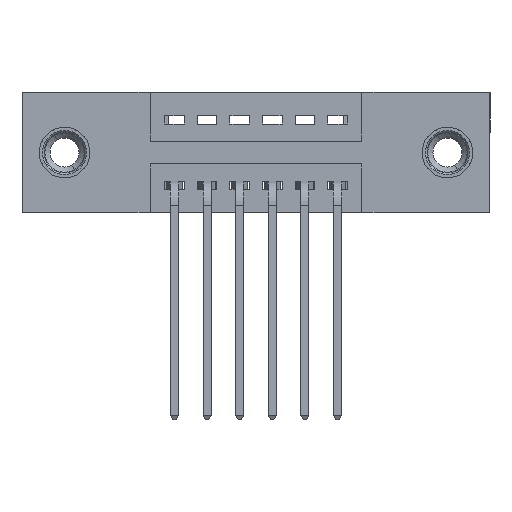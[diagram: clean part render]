
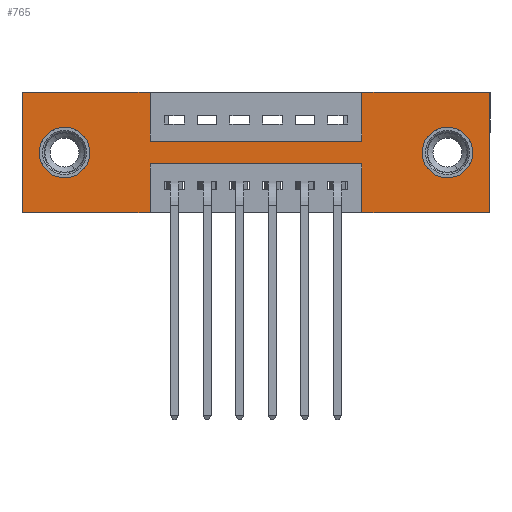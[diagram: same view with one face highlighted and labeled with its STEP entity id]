
A CAD part, front view. The second image highlights one B-rep face of the part: STEP entity #765.
In plain terms, the highlighted planar face has unit normal (0, -1, 0).
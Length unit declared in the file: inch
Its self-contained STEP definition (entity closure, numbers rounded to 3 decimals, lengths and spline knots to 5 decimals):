
#94 = EDGE_CURVE ( 'NONE', #12431, #1138, #12503, .T. ) ;
#183 = VECTOR ( 'NONE', #4928, 39.37008 ) ;
#296 = FACE_BOUND ( 'NONE', #9028, .T. ) ;
#588 = CIRCLE ( 'NONE', #4915, 0.078 ) ;
#644 = CARTESIAN_POINT ( 'NONE',  ( 0.13, 0., -0.107 ) ) ;
#658 = ORIENTED_EDGE ( 'NONE', *, *, #10039, .F. ) ;
#765 = ADVANCED_FACE ( 'NONE', ( #4771, #296, #13489 ), #11098, .T. ) ;
#838 = VERTEX_POINT ( 'NONE', #5530 ) ;
#1138 = VERTEX_POINT ( 'NONE', #4485 ) ;
#1227 = CARTESIAN_POINT ( 'NONE',  ( 0.3925, 0., -0.22 ) ) ;
#1370 = ORIENTED_EDGE ( 'NONE', *, *, #6849, .F. ) ;
#1428 = VECTOR ( 'NONE', #5903, 39.37008 ) ;
#1485 = VERTEX_POINT ( 'NONE', #1607 ) ;
#1607 = CARTESIAN_POINT ( 'NONE',  ( 0.3925, 0., -0.37 ) ) ;
#1695 = CARTESIAN_POINT ( 'NONE',  ( 0., 0., 0. ) ) ;
#1705 = LINE ( 'NONE', #1920, #8583 ) ;
#1823 = ORIENTED_EDGE ( 'NONE', *, *, #6230, .F. ) ;
#1887 = CARTESIAN_POINT ( 'NONE',  ( 0.13, 0., -0.185 ) ) ;
#1916 = ORIENTED_EDGE ( 'NONE', *, *, #2650, .T. ) ;
#1920 = CARTESIAN_POINT ( 'NONE',  ( 0.3925, 0., -0.15 ) ) ;
#1935 = VECTOR ( 'NONE', #2283, 39.37008 ) ;
#2012 = CARTESIAN_POINT ( 'NONE',  ( 0., 0., 0. ) ) ;
#2047 = CARTESIAN_POINT ( 'NONE',  ( 0.3925, 0., 0. ) ) ;
#2082 = CARTESIAN_POINT ( 'NONE',  ( 0., 0., 0. ) ) ;
#2233 = AXIS2_PLACEMENT_3D ( 'NONE', #7778, #4527, #12016 ) ;
#2283 = DIRECTION ( 'NONE',  ( 1., 0., 0. ) ) ;
#2321 = VECTOR ( 'NONE', #12269, 39.37008 ) ;
#2354 = VERTEX_POINT ( 'NONE', #5692 ) ;
#2363 = DIRECTION ( 'NONE',  ( -1., 0., 0. ) ) ;
#2560 = EDGE_LOOP ( 'NONE', ( #4301, #13436, #2651, #9678, #12162, #1823, #13720, #3026, #12351, #4077, #658, #1370 ) ) ;
#2614 = VERTEX_POINT ( 'NONE', #6707 ) ;
#2650 = EDGE_CURVE ( 'NONE', #10516, #6219, #588, .T. ) ;
#2651 = ORIENTED_EDGE ( 'NONE', *, *, #5780, .F. ) ;
#2665 = DIRECTION ( 'NONE',  ( 0., 0., 1. ) ) ;
#2971 = ORIENTED_EDGE ( 'NONE', *, *, #10768, .T. ) ;
#3026 = ORIENTED_EDGE ( 'NONE', *, *, #8182, .F. ) ;
#3046 = EDGE_CURVE ( 'NONE', #6951, #1485, #12585, .T. ) ;
#3249 = CARTESIAN_POINT ( 'NONE',  ( 0.3925, 0., -0.22 ) ) ;
#3559 = VERTEX_POINT ( 'NONE', #11444 ) ;
#3648 = LINE ( 'NONE', #7883, #11912 ) ;
#4024 = VERTEX_POINT ( 'NONE', #13758 ) ;
#4077 = ORIENTED_EDGE ( 'NONE', *, *, #7554, .F. ) ;
#4165 = CARTESIAN_POINT ( 'NONE',  ( 1.435, 0., 0. ) ) ;
#4234 = DIRECTION ( 'NONE',  ( 1., 0., 0. ) ) ;
#4301 = ORIENTED_EDGE ( 'NONE', *, *, #3046, .F. ) ;
#4451 = CARTESIAN_POINT ( 'NONE',  ( 1.305, 0., -0.107 ) ) ;
#4457 = VERTEX_POINT ( 'NONE', #2082 ) ;
#4485 = CARTESIAN_POINT ( 'NONE',  ( 0.13, 0., -0.263 ) ) ;
#4527 = DIRECTION ( 'NONE',  ( 0., -1., 0. ) ) ;
#4605 = CARTESIAN_POINT ( 'NONE',  ( 0., 0., 0. ) ) ;
#4749 = AXIS2_PLACEMENT_3D ( 'NONE', #12182, #8844, #5546 ) ;
#4771 = FACE_BOUND ( 'NONE', #10620, .T. ) ;
#4864 = CIRCLE ( 'NONE', #4749, 0.078 ) ;
#4915 = AXIS2_PLACEMENT_3D ( 'NONE', #13751, #6029, #13695 ) ;
#4928 = DIRECTION ( 'NONE',  ( 1., 0., 0. ) ) ;
#5133 = VECTOR ( 'NONE', #6465, 39.37008 ) ;
#5167 = EDGE_CURVE ( 'NONE', #2614, #4024, #11950, .T. ) ;
#5211 = LINE ( 'NONE', #4605, #1935 ) ;
#5275 = CIRCLE ( 'NONE', #9365, 0.078 ) ;
#5514 = LINE ( 'NONE', #1695, #183 ) ;
#5530 = CARTESIAN_POINT ( 'NONE',  ( 1.0425, 0., -0.15 ) ) ;
#5546 = DIRECTION ( 'NONE',  ( 0., 0., 1. ) ) ;
#5692 = CARTESIAN_POINT ( 'NONE',  ( 1.0425, 0., -0.37 ) ) ;
#5780 = EDGE_CURVE ( 'NONE', #2354, #13346, #12097, .T. ) ;
#5903 = DIRECTION ( 'NONE',  ( 0., 0., 1. ) ) ;
#6029 = DIRECTION ( 'NONE',  ( 0., 1., 0. ) ) ;
#6170 = EDGE_CURVE ( 'NONE', #1138, #12431, #4864, .T. ) ;
#6219 = VERTEX_POINT ( 'NONE', #4451 ) ;
#6230 = EDGE_CURVE ( 'NONE', #8744, #9569, #5211, .T. ) ;
#6450 = VECTOR ( 'NONE', #7791, 39.37008 ) ;
#6465 = DIRECTION ( 'NONE',  ( 0., 0., 1. ) ) ;
#6500 = VERTEX_POINT ( 'NONE', #12786 ) ;
#6707 = CARTESIAN_POINT ( 'NONE',  ( 0.3925, 0., 0. ) ) ;
#6849 = EDGE_CURVE ( 'NONE', #1485, #6500, #3648, .T. ) ;
#6951 = VERTEX_POINT ( 'NONE', #3249 ) ;
#7129 = VECTOR ( 'NONE', #11773, 39.37008 ) ;
#7184 = CARTESIAN_POINT ( 'NONE',  ( 1.0425, 0., 0. ) ) ;
#7331 = CARTESIAN_POINT ( 'NONE',  ( 0.3925, 0., -0.37 ) ) ;
#7434 = EDGE_CURVE ( 'NONE', #13346, #6951, #10318, .T. ) ;
#7473 = LINE ( 'NONE', #13347, #2321 ) ;
#7554 = EDGE_CURVE ( 'NONE', #4457, #2614, #5514, .T. ) ;
#7778 = CARTESIAN_POINT ( 'NONE',  ( 0., 0., -0.37 ) ) ;
#7791 = DIRECTION ( 'NONE',  ( 0., 0., -1. ) ) ;
#7883 = CARTESIAN_POINT ( 'NONE',  ( 0., 0., -0.37 ) ) ;
#7947 = CARTESIAN_POINT ( 'NONE',  ( 1.435, 0., 0. ) ) ;
#8096 = VECTOR ( 'NONE', #9911, 39.37008 ) ;
#8182 = EDGE_CURVE ( 'NONE', #4024, #838, #1705, .T. ) ;
#8235 = LINE ( 'NONE', #7184, #9094 ) ;
#8583 = VECTOR ( 'NONE', #4234, 39.37008 ) ;
#8744 = VERTEX_POINT ( 'NONE', #12325 ) ;
#8844 = DIRECTION ( 'NONE',  ( 0., 1., 0. ) ) ;
#8862 = EDGE_CURVE ( 'NONE', #838, #8744, #8235, .T. ) ;
#9028 = EDGE_LOOP ( 'NONE', ( #12645, #10441 ) ) ;
#9094 = VECTOR ( 'NONE', #2665, 39.37008 ) ;
#9220 = CARTESIAN_POINT ( 'NONE',  ( 1.0425, 0., -0.37 ) ) ;
#9316 = VECTOR ( 'NONE', #9525, 39.37008 ) ;
#9365 = AXIS2_PLACEMENT_3D ( 'NONE', #11651, #9475, #9372 ) ;
#9372 = DIRECTION ( 'NONE',  ( 0., 0., -1. ) ) ;
#9475 = DIRECTION ( 'NONE',  ( 0., 1., 0. ) ) ;
#9525 = DIRECTION ( 'NONE',  ( 0., 0., -1. ) ) ;
#9569 = VERTEX_POINT ( 'NONE', #4165 ) ;
#9587 = CARTESIAN_POINT ( 'NONE',  ( 1.0425, 0., -0.22 ) ) ;
#9678 = ORIENTED_EDGE ( 'NONE', *, *, #13929, .F. ) ;
#9911 = DIRECTION ( 'NONE',  ( -1., 0., 0. ) ) ;
#10039 = EDGE_CURVE ( 'NONE', #6500, #4457, #14212, .T. ) ;
#10318 = LINE ( 'NONE', #1227, #8096 ) ;
#10441 = ORIENTED_EDGE ( 'NONE', *, *, #6170, .T. ) ;
#10488 = AXIS2_PLACEMENT_3D ( 'NONE', #1887, #13277, #13412 ) ;
#10516 = VERTEX_POINT ( 'NONE', #10960 ) ;
#10620 = EDGE_LOOP ( 'NONE', ( #2971, #1916 ) ) ;
#10768 = EDGE_CURVE ( 'NONE', #6219, #10516, #5275, .T. ) ;
#10960 = CARTESIAN_POINT ( 'NONE',  ( 1.305, 0., -0.263 ) ) ;
#11098 = PLANE ( 'NONE',  #2233 ) ;
#11444 = CARTESIAN_POINT ( 'NONE',  ( 1.435, 0., -0.37 ) ) ;
#11651 = CARTESIAN_POINT ( 'NONE',  ( 1.305, 0., -0.185 ) ) ;
#11773 = DIRECTION ( 'NONE',  ( 0., 0., -1. ) ) ;
#11912 = VECTOR ( 'NONE', #2363, 39.37008 ) ;
#11950 = LINE ( 'NONE', #2047, #7129 ) ;
#12016 = DIRECTION ( 'NONE',  ( 0., 0., -1. ) ) ;
#12097 = LINE ( 'NONE', #9220, #1428 ) ;
#12158 = LINE ( 'NONE', #7947, #6450 ) ;
#12162 = ORIENTED_EDGE ( 'NONE', *, *, #12655, .F. ) ;
#12182 = CARTESIAN_POINT ( 'NONE',  ( 0.13, 0., -0.185 ) ) ;
#12269 = DIRECTION ( 'NONE',  ( -1., 0., 0. ) ) ;
#12325 = CARTESIAN_POINT ( 'NONE',  ( 1.0425, 0., 0. ) ) ;
#12351 = ORIENTED_EDGE ( 'NONE', *, *, #5167, .F. ) ;
#12431 = VERTEX_POINT ( 'NONE', #644 ) ;
#12503 = CIRCLE ( 'NONE', #10488, 0.078 ) ;
#12585 = LINE ( 'NONE', #7331, #9316 ) ;
#12645 = ORIENTED_EDGE ( 'NONE', *, *, #94, .T. ) ;
#12655 = EDGE_CURVE ( 'NONE', #9569, #3559, #12158, .T. ) ;
#12786 = CARTESIAN_POINT ( 'NONE',  ( 0., 0., -0.37 ) ) ;
#13277 = DIRECTION ( 'NONE',  ( 0., 1., 0. ) ) ;
#13346 = VERTEX_POINT ( 'NONE', #9587 ) ;
#13347 = CARTESIAN_POINT ( 'NONE',  ( 0., 0., -0.37 ) ) ;
#13412 = DIRECTION ( 'NONE',  ( 0., 0., 1. ) ) ;
#13436 = ORIENTED_EDGE ( 'NONE', *, *, #7434, .F. ) ;
#13489 = FACE_OUTER_BOUND ( 'NONE', #2560, .T. ) ;
#13695 = DIRECTION ( 'NONE',  ( 0., 0., -1. ) ) ;
#13720 = ORIENTED_EDGE ( 'NONE', *, *, #8862, .F. ) ;
#13751 = CARTESIAN_POINT ( 'NONE',  ( 1.305, 0., -0.185 ) ) ;
#13758 = CARTESIAN_POINT ( 'NONE',  ( 0.3925, 0., -0.15 ) ) ;
#13929 = EDGE_CURVE ( 'NONE', #3559, #2354, #7473, .T. ) ;
#14212 = LINE ( 'NONE', #2012, #5133 ) ;
